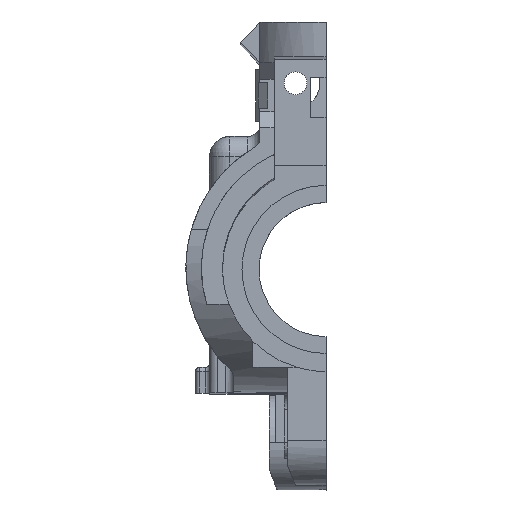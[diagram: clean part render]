
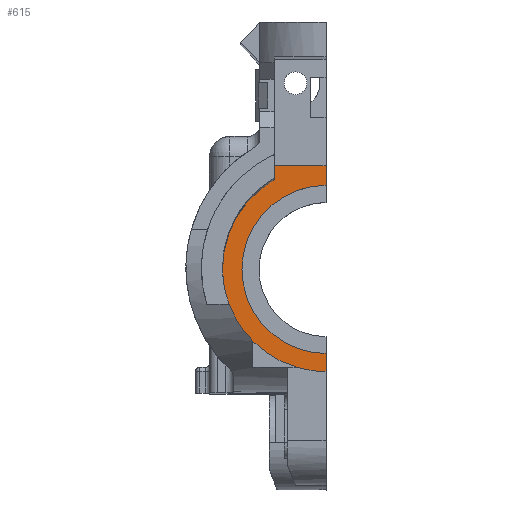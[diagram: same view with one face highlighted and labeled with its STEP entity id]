
A CAD part, top view. The second image highlights one B-rep face of the part: STEP entity #615.
In plain terms, the highlighted planar face has unit normal (0, 0, 1).
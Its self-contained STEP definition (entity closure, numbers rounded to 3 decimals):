
#34 = CARTESIAN_POINT ( 'NONE',  ( -6.4, 12.75, -113. ) ) ;
#63 = VERTEX_POINT ( 'NONE', #2987 ) ;
#187 = VERTEX_POINT ( 'NONE', #4109 ) ;
#232 = CARTESIAN_POINT ( 'NONE',  ( -10.35, 0., -113. ) ) ;
#455 = CARTESIAN_POINT ( 'NONE',  ( 0., -15.25, -113. ) ) ;
#615 = ADVANCED_FACE ( 'NONE', ( #10813 ), #7854, .F. ) ;
#987 = CARTESIAN_POINT ( 'NONE',  ( -12., -4.308, -113. ) ) ;
#1260 = CARTESIAN_POINT ( 'NONE',  ( 6.4, 12.75, -113. ) ) ;
#1262 = CARTESIAN_POINT ( 'NONE',  ( 0., -10.35, -113. ) ) ;
#1285 = EDGE_CURVE ( 'NONE', #7390, #3299, #3814, .T. ) ;
#1331 = DIRECTION ( 'NONE',  ( 0., -1., 0. ) ) ;
#1346 = DIRECTION ( 'NONE',  ( 0., 0., 1. ) ) ;
#1813 = VECTOR ( 'NONE', #12108, 1000. ) ;
#2058 = CARTESIAN_POINT ( 'NONE',  ( 0., 0., -113. ) ) ;
#2195 = EDGE_CURVE ( 'NONE', #63, #3738, #9089, .T. ) ;
#2644 = DIRECTION ( 'NONE',  ( 0., 0., -1. ) ) ;
#2834 = EDGE_CURVE ( 'NONE', #12572, #5494, #11109, .T. ) ;
#2987 = CARTESIAN_POINT ( 'NONE',  ( -6.4, 11.027, -113. ) ) ;
#3078 = DIRECTION ( 'NONE',  ( -1., 0., 0. ) ) ;
#3109 = CARTESIAN_POINT ( 'NONE',  ( -12., -15.25, -113. ) ) ;
#3299 = VERTEX_POINT ( 'NONE', #455 ) ;
#3567 = EDGE_CURVE ( 'NONE', #12572, #187, #12669, .T. ) ;
#3700 = ORIENTED_EDGE ( 'NONE', *, *, #7975, .F. ) ;
#3738 = VERTEX_POINT ( 'NONE', #12301 ) ;
#3814 = LINE ( 'NONE', #10296, #6492 ) ;
#4058 = CIRCLE ( 'NONE', #4652, 12.75 ) ;
#4109 = CARTESIAN_POINT ( 'NONE',  ( 0., 10.35, -113. ) ) ;
#4148 = EDGE_LOOP ( 'NONE', ( #5822, #4651, #11391, #11690, #12730, #7303, #6077, #11421, #11731, #5707, #3700 ) ) ;
#4243 = VECTOR ( 'NONE', #1331, 1000. ) ;
#4384 = CARTESIAN_POINT ( 'NONE',  ( -6.4, 12.75, -113. ) ) ;
#4479 = CARTESIAN_POINT ( 'NONE',  ( 0., 12.75, -113. ) ) ;
#4651 = ORIENTED_EDGE ( 'NONE', *, *, #2834, .T. ) ;
#4652 = AXIS2_PLACEMENT_3D ( 'NONE', #2058, #9145, #3078 ) ;
#4879 = DIRECTION ( 'NONE',  ( -1., 0., 0. ) ) ;
#4997 = CARTESIAN_POINT ( 'NONE',  ( -10.5, -7.233, -113. ) ) ;
#5103 = DIRECTION ( 'NONE',  ( 1., 0., 0. ) ) ;
#5176 = EDGE_CURVE ( 'NONE', #3738, #9612, #4058, .T. ) ;
#5268 = VERTEX_POINT ( 'NONE', #1262 ) ;
#5299 = CIRCLE ( 'NONE', #6615, 10.35 ) ;
#5477 = CARTESIAN_POINT ( 'NONE',  ( 0., 0., -113. ) ) ;
#5494 = VERTEX_POINT ( 'NONE', #4384 ) ;
#5527 = DIRECTION ( 'NONE',  ( -1., 0., 0. ) ) ;
#5707 = ORIENTED_EDGE ( 'NONE', *, *, #10788, .F. ) ;
#5816 = EDGE_CURVE ( 'NONE', #7651, #9612, #6548, .T. ) ;
#5822 = ORIENTED_EDGE ( 'NONE', *, *, #3567, .F. ) ;
#5979 = AXIS2_PLACEMENT_3D ( 'NONE', #8539, #8591, #10596 ) ;
#6077 = ORIENTED_EDGE ( 'NONE', *, *, #8362, .T. ) ;
#6252 = DIRECTION ( 'NONE',  ( 1., 0., 0. ) ) ;
#6492 = VECTOR ( 'NONE', #5103, 1000. ) ;
#6541 = LINE ( 'NONE', #11604, #7038 ) ;
#6548 = CIRCLE ( 'NONE', #6591, 5. ) ;
#6591 = AXIS2_PLACEMENT_3D ( 'NONE', #9702, #2644, #8900 ) ;
#6615 = AXIS2_PLACEMENT_3D ( 'NONE', #12689, #7597, #8631 ) ;
#7038 = VECTOR ( 'NONE', #11647, 1000. ) ;
#7303 = ORIENTED_EDGE ( 'NONE', *, *, #5816, .F. ) ;
#7390 = VERTEX_POINT ( 'NONE', #3109 ) ;
#7597 = DIRECTION ( 'NONE',  ( 0., 0., 1. ) ) ;
#7651 = VERTEX_POINT ( 'NONE', #9658 ) ;
#7854 = PLANE ( 'NONE',  #9780 ) ;
#7941 = DIRECTION ( 'NONE',  ( 0., 0., -1. ) ) ;
#7951 = EDGE_CURVE ( 'NONE', #5494, #63, #7995, .T. ) ;
#7975 = EDGE_CURVE ( 'NONE', #187, #10286, #5299, .T. ) ;
#7995 = LINE ( 'NONE', #34, #12789 ) ;
#8297 = CARTESIAN_POINT ( 'NONE',  ( 0., 0., -113. ) ) ;
#8362 = EDGE_CURVE ( 'NONE', #7651, #7390, #8788, .T. ) ;
#8524 = EDGE_CURVE ( 'NONE', #5268, #3299, #6541, .T. ) ;
#8525 = AXIS2_PLACEMENT_3D ( 'NONE', #8297, #1346, #6252 ) ;
#8539 = CARTESIAN_POINT ( 'NONE',  ( 0., 0., -113. ) ) ;
#8591 = DIRECTION ( 'NONE',  ( 0., 0., 1. ) ) ;
#8631 = DIRECTION ( 'NONE',  ( 1., 0., 0. ) ) ;
#8788 = LINE ( 'NONE', #987, #1813 ) ;
#8900 = DIRECTION ( 'NONE',  ( -1., 0., 0. ) ) ;
#8907 = DIRECTION ( 'NONE',  ( 0., -1., 0. ) ) ;
#9089 = CIRCLE ( 'NONE', #5979, 12.75 ) ;
#9145 = DIRECTION ( 'NONE',  ( 0., 0., 1. ) ) ;
#9523 = CIRCLE ( 'NONE', #8525, 10.35 ) ;
#9612 = VERTEX_POINT ( 'NONE', #4997 ) ;
#9658 = CARTESIAN_POINT ( 'NONE',  ( -12., -9.75, -113. ) ) ;
#9702 = CARTESIAN_POINT ( 'NONE',  ( -7.143, -10.938, -113. ) ) ;
#9780 = AXIS2_PLACEMENT_3D ( 'NONE', #13030, #7941, #4879 ) ;
#9809 = VECTOR ( 'NONE', #5527, 1000. ) ;
#10286 = VERTEX_POINT ( 'NONE', #232 ) ;
#10296 = CARTESIAN_POINT ( 'NONE',  ( -12., -15.25, -113. ) ) ;
#10596 = DIRECTION ( 'NONE',  ( -1., 0., 0. ) ) ;
#10788 = EDGE_CURVE ( 'NONE', #10286, #5268, #9523, .T. ) ;
#10813 = FACE_OUTER_BOUND ( 'NONE', #4148, .T. ) ;
#11109 = LINE ( 'NONE', #1260, #9809 ) ;
#11391 = ORIENTED_EDGE ( 'NONE', *, *, #7951, .T. ) ;
#11421 = ORIENTED_EDGE ( 'NONE', *, *, #1285, .T. ) ;
#11604 = CARTESIAN_POINT ( 'NONE',  ( 0., 0., -113. ) ) ;
#11647 = DIRECTION ( 'NONE',  ( 0., -1., 0. ) ) ;
#11690 = ORIENTED_EDGE ( 'NONE', *, *, #2195, .T. ) ;
#11731 = ORIENTED_EDGE ( 'NONE', *, *, #8524, .F. ) ;
#12108 = DIRECTION ( 'NONE',  ( 0., -1., 0. ) ) ;
#12301 = CARTESIAN_POINT ( 'NONE',  ( -12.75, 0., -113. ) ) ;
#12572 = VERTEX_POINT ( 'NONE', #4479 ) ;
#12669 = LINE ( 'NONE', #5477, #4243 ) ;
#12689 = CARTESIAN_POINT ( 'NONE',  ( 0., 0., -113. ) ) ;
#12730 = ORIENTED_EDGE ( 'NONE', *, *, #5176, .T. ) ;
#12789 = VECTOR ( 'NONE', #8907, 1000. ) ;
#13030 = CARTESIAN_POINT ( 'NONE',  ( 0., 0., -113. ) ) ;
